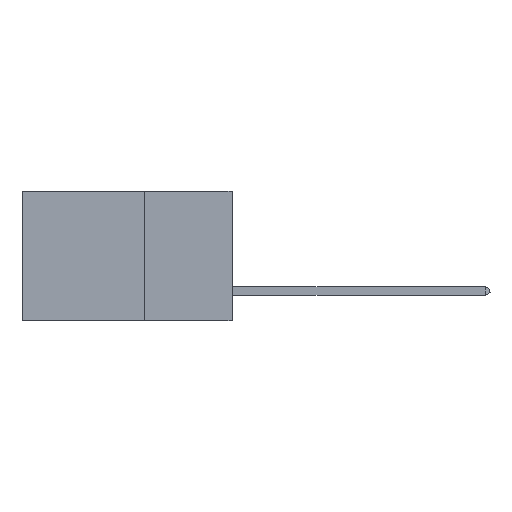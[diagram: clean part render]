
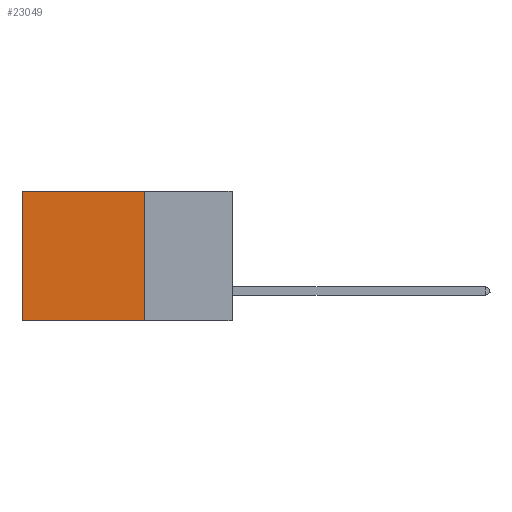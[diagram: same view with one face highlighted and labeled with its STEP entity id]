
A CAD part, left-side view. The second image highlights one B-rep face of the part: STEP entity #23049.
In plain terms, the highlighted planar face has unit normal (-1, 0, 0).
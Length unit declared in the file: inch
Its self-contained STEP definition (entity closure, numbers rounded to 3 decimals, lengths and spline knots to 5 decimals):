
#795 = CARTESIAN_POINT ( 'NONE',  ( 0.2875, 0.25, 0. ) ) ;
#1168 = DIRECTION ( 'NONE',  ( 0., 0., -1. ) ) ;
#1222 = CARTESIAN_POINT ( 'NONE',  ( 0.2875, 0.25, -0.37 ) ) ;
#1494 = PLANE ( 'NONE',  #16058 ) ;
#2039 = CARTESIAN_POINT ( 'NONE',  ( 0.2875, 0.25, -0.37 ) ) ;
#2473 = DIRECTION ( 'NONE',  ( 0., 1., 0. ) ) ;
#3010 = DIRECTION ( 'NONE',  ( 1., 0., 0. ) ) ;
#3230 = DIRECTION ( 'NONE',  ( 0., 0., -1. ) ) ;
#3390 = ORIENTED_EDGE ( 'NONE', *, *, #22580, .F. ) ;
#4396 = VERTEX_POINT ( 'NONE', #2039 ) ;
#5172 = EDGE_LOOP ( 'NONE', ( #7605, #3390, #8174, #10030 ) ) ;
#7605 = ORIENTED_EDGE ( 'NONE', *, *, #11944, .T. ) ;
#7825 = LINE ( 'NONE', #14241, #22303 ) ;
#7983 = DIRECTION ( 'NONE',  ( 0., 0., -1. ) ) ;
#8174 = ORIENTED_EDGE ( 'NONE', *, *, #19448, .F. ) ;
#8554 = VERTEX_POINT ( 'NONE', #795 ) ;
#10030 = ORIENTED_EDGE ( 'NONE', *, *, #11870, .T. ) ;
#10112 = VECTOR ( 'NONE', #2473, 39.37008 ) ;
#10797 = CARTESIAN_POINT ( 'NONE',  ( 0.2875, 0.6, -0.37 ) ) ;
#11324 = VERTEX_POINT ( 'NONE', #18158 ) ;
#11870 = EDGE_CURVE ( 'NONE', #8554, #11324, #15000, .T. ) ;
#11944 = EDGE_CURVE ( 'NONE', #11324, #14770, #14690, .T. ) ;
#14241 = CARTESIAN_POINT ( 'NONE',  ( 0.2875, 0.25, 0. ) ) ;
#14265 = CARTESIAN_POINT ( 'NONE',  ( 0.2875, 0.25, 0. ) ) ;
#14690 = LINE ( 'NONE', #18844, #18341 ) ;
#14770 = VERTEX_POINT ( 'NONE', #10797 ) ;
#15000 = LINE ( 'NONE', #17102, #10112 ) ;
#15828 = DIRECTION ( 'NONE',  ( 0., 1., 0. ) ) ;
#16058 = AXIS2_PLACEMENT_3D ( 'NONE', #14265, #3010, #1168 ) ;
#17102 = CARTESIAN_POINT ( 'NONE',  ( 0.2875, 0.25, 0. ) ) ;
#18158 = CARTESIAN_POINT ( 'NONE',  ( 0.2875, 0.6, 0. ) ) ;
#18341 = VECTOR ( 'NONE', #7983, 39.37008 ) ;
#18496 = LINE ( 'NONE', #1222, #19045 ) ;
#18844 = CARTESIAN_POINT ( 'NONE',  ( 0.2875, 0.6, 0. ) ) ;
#19045 = VECTOR ( 'NONE', #15828, 39.37008 ) ;
#19448 = EDGE_CURVE ( 'NONE', #8554, #4396, #7825, .T. ) ;
#22169 = FACE_OUTER_BOUND ( 'NONE', #5172, .T. ) ;
#22303 = VECTOR ( 'NONE', #3230, 39.37008 ) ;
#22580 = EDGE_CURVE ( 'NONE', #4396, #14770, #18496, .T. ) ;
#23049 = ADVANCED_FACE ( 'NONE', ( #22169 ), #1494, .F. ) ;
